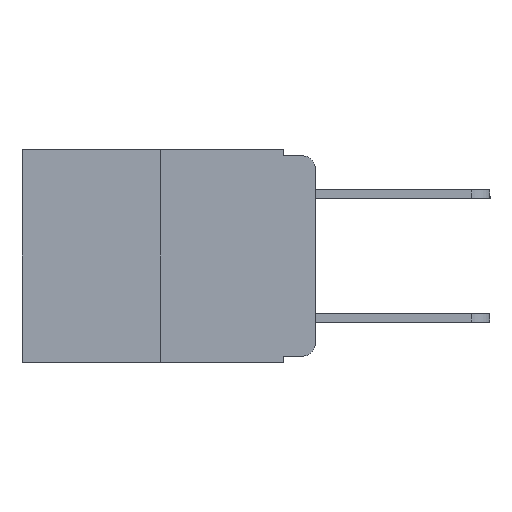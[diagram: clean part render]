
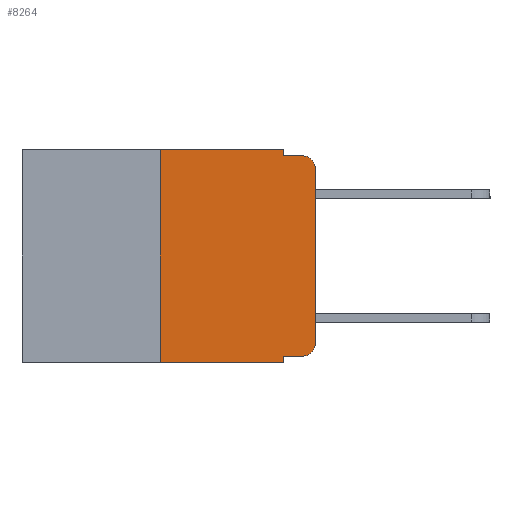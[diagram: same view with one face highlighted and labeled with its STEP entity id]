
A CAD part, left-side view. The second image highlights one B-rep face of the part: STEP entity #8264.
In plain terms, the highlighted planar face has unit normal (-1, 0, 0).
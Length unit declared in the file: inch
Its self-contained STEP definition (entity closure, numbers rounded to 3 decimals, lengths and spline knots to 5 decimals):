
#19 = PLANE ( 'NONE',  #15869 ) ;
#264 = EDGE_CURVE ( 'NONE', #9095, #7282, #10863, .T. ) ;
#304 = EDGE_CURVE ( 'NONE', #713, #9192, #16703, .T. ) ;
#430 = CARTESIAN_POINT ( 'NONE',  ( 0., 0., 0. ) ) ;
#713 = VERTEX_POINT ( 'NONE', #3043 ) ;
#1132 = ORIENTED_EDGE ( 'NONE', *, *, #3417, .F. ) ;
#1350 = CARTESIAN_POINT ( 'NONE',  ( 0., 0.051, 0. ) ) ;
#1360 = CARTESIAN_POINT ( 'NONE',  ( 0., 0., -0.313 ) ) ;
#2074 = VERTEX_POINT ( 'NONE', #7991 ) ;
#2124 = VECTOR ( 'NONE', #17701, 39.37008 ) ;
#2296 = CARTESIAN_POINT ( 'NONE',  ( 0., 0.051, -0.333 ) ) ;
#2413 = CARTESIAN_POINT ( 'NONE',  ( 0., 0.473, -0.343 ) ) ;
#2818 = CARTESIAN_POINT ( 'NONE',  ( 0., 0.02, -0.313 ) ) ;
#3038 = ORIENTED_EDGE ( 'NONE', *, *, #17013, .T. ) ;
#3043 = CARTESIAN_POINT ( 'NONE',  ( 0., 0.051, 0. ) ) ;
#3101 = DIRECTION ( 'NONE',  ( 0., 0., -1. ) ) ;
#3148 = CARTESIAN_POINT ( 'NONE',  ( 0., 0.02, -0.03 ) ) ;
#3299 = ORIENTED_EDGE ( 'NONE', *, *, #13597, .T. ) ;
#3342 = VECTOR ( 'NONE', #10723, 39.37008 ) ;
#3372 = CIRCLE ( 'NONE', #15613, 0.02 ) ;
#3417 = EDGE_CURVE ( 'NONE', #2074, #4568, #15898, .T. ) ;
#3561 = ORIENTED_EDGE ( 'NONE', *, *, #16989, .F. ) ;
#3886 = DIRECTION ( 'NONE',  ( 0., 0., 1. ) ) ;
#4106 = ORIENTED_EDGE ( 'NONE', *, *, #304, .F. ) ;
#4255 = AXIS2_PLACEMENT_3D ( 'NONE', #2818, #16588, #7981 ) ;
#4278 = VECTOR ( 'NONE', #17465, 39.37008 ) ;
#4317 = EDGE_CURVE ( 'NONE', #13259, #12746, #12816, .T. ) ;
#4568 = VERTEX_POINT ( 'NONE', #12547 ) ;
#4885 = DIRECTION ( 'NONE',  ( 0., 0., -1. ) ) ;
#5008 = CARTESIAN_POINT ( 'NONE',  ( 0., 0., -0.03 ) ) ;
#5282 = CARTESIAN_POINT ( 'NONE',  ( 0., 0.473, 0. ) ) ;
#6069 = VECTOR ( 'NONE', #16508, 39.37008 ) ;
#6115 = VECTOR ( 'NONE', #3886, 39.37008 ) ;
#6199 = EDGE_CURVE ( 'NONE', #9095, #13259, #12486, .T. ) ;
#7176 = CARTESIAN_POINT ( 'NONE',  ( 0., 0.051, -0.343 ) ) ;
#7282 = VERTEX_POINT ( 'NONE', #7176 ) ;
#7981 = DIRECTION ( 'NONE',  ( 0., 0., -1. ) ) ;
#7991 = CARTESIAN_POINT ( 'NONE',  ( 0., 0.25, -0.343 ) ) ;
#8264 = ADVANCED_FACE ( 'NONE', ( #8967 ), #19, .F. ) ;
#8275 = EDGE_LOOP ( 'NONE', ( #3038, #19271, #3561, #4106, #17378, #1132, #3299, #12570, #13045, #9402 ) ) ;
#8291 = VECTOR ( 'NONE', #8906, 39.37008 ) ;
#8906 = DIRECTION ( 'NONE',  ( 0., -1., 0. ) ) ;
#8967 = FACE_OUTER_BOUND ( 'NONE', #8275, .T. ) ;
#9095 = VERTEX_POINT ( 'NONE', #2296 ) ;
#9192 = VERTEX_POINT ( 'NONE', #15327 ) ;
#9402 = ORIENTED_EDGE ( 'NONE', *, *, #4317, .T. ) ;
#10723 = DIRECTION ( 'NONE',  ( 0., 0., 1. ) ) ;
#10863 = LINE ( 'NONE', #1350, #14354 ) ;
#10971 = CARTESIAN_POINT ( 'NONE',  ( 0., 0.051, -0.333 ) ) ;
#11698 = DIRECTION ( 'NONE',  ( 1., 0., 0. ) ) ;
#11775 = CARTESIAN_POINT ( 'NONE',  ( 0., 0.473, 0. ) ) ;
#12486 = LINE ( 'NONE', #10971, #8291 ) ;
#12547 = CARTESIAN_POINT ( 'NONE',  ( 0., 0.25, 0. ) ) ;
#12570 = ORIENTED_EDGE ( 'NONE', *, *, #264, .F. ) ;
#12746 = VERTEX_POINT ( 'NONE', #1360 ) ;
#12816 = CIRCLE ( 'NONE', #4255, 0.02 ) ;
#12957 = LINE ( 'NONE', #5282, #4278 ) ;
#13018 = VECTOR ( 'NONE', #15430, 39.37008 ) ;
#13045 = ORIENTED_EDGE ( 'NONE', *, *, #6199, .T. ) ;
#13259 = VERTEX_POINT ( 'NONE', #16144 ) ;
#13276 = DIRECTION ( 'NONE',  ( 0., 0., -1. ) ) ;
#13597 = EDGE_CURVE ( 'NONE', #2074, #7282, #14463, .T. ) ;
#14172 = CARTESIAN_POINT ( 'NONE',  ( 0., 0.25, 0. ) ) ;
#14354 = VECTOR ( 'NONE', #3101, 39.37008 ) ;
#14386 = DIRECTION ( 'NONE',  ( -1., 0., 0. ) ) ;
#14463 = LINE ( 'NONE', #2413, #6069 ) ;
#14502 = LINE ( 'NONE', #430, #6115 ) ;
#14899 = EDGE_CURVE ( 'NONE', #15853, #15335, #3372, .T. ) ;
#14929 = LINE ( 'NONE', #16315, #2124 ) ;
#15327 = CARTESIAN_POINT ( 'NONE',  ( 0., 0.051, -0.01 ) ) ;
#15335 = VERTEX_POINT ( 'NONE', #17743 ) ;
#15430 = DIRECTION ( 'NONE',  ( 0., 0., -1. ) ) ;
#15613 = AXIS2_PLACEMENT_3D ( 'NONE', #3148, #14386, #4885 ) ;
#15853 = VERTEX_POINT ( 'NONE', #5008 ) ;
#15869 = AXIS2_PLACEMENT_3D ( 'NONE', #11775, #11698, #13276 ) ;
#15898 = LINE ( 'NONE', #14172, #3342 ) ;
#16144 = CARTESIAN_POINT ( 'NONE',  ( 0., 0.02, -0.333 ) ) ;
#16315 = CARTESIAN_POINT ( 'NONE',  ( 0., 0.051, -0.01 ) ) ;
#16508 = DIRECTION ( 'NONE',  ( 0., -1., 0. ) ) ;
#16588 = DIRECTION ( 'NONE',  ( -1., 0., 0. ) ) ;
#16703 = LINE ( 'NONE', #17238, #13018 ) ;
#16911 = EDGE_CURVE ( 'NONE', #4568, #713, #12957, .T. ) ;
#16989 = EDGE_CURVE ( 'NONE', #9192, #15335, #14929, .T. ) ;
#17013 = EDGE_CURVE ( 'NONE', #12746, #15853, #14502, .T. ) ;
#17238 = CARTESIAN_POINT ( 'NONE',  ( 0., 0.051, 0. ) ) ;
#17378 = ORIENTED_EDGE ( 'NONE', *, *, #16911, .F. ) ;
#17465 = DIRECTION ( 'NONE',  ( 0., -1., 0. ) ) ;
#17701 = DIRECTION ( 'NONE',  ( 0., -1., 0. ) ) ;
#17743 = CARTESIAN_POINT ( 'NONE',  ( 0., 0.02, -0.01 ) ) ;
#19271 = ORIENTED_EDGE ( 'NONE', *, *, #14899, .T. ) ;
